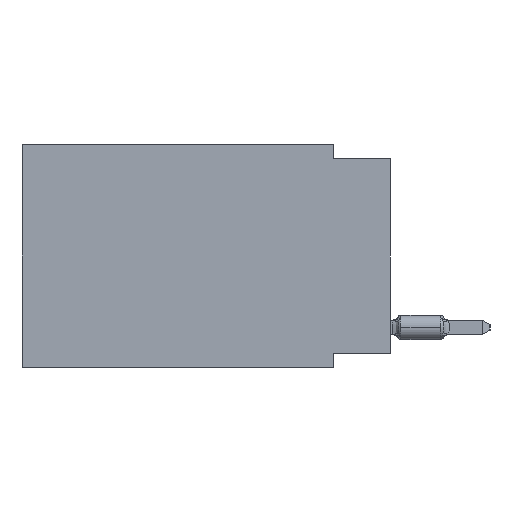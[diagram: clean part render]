
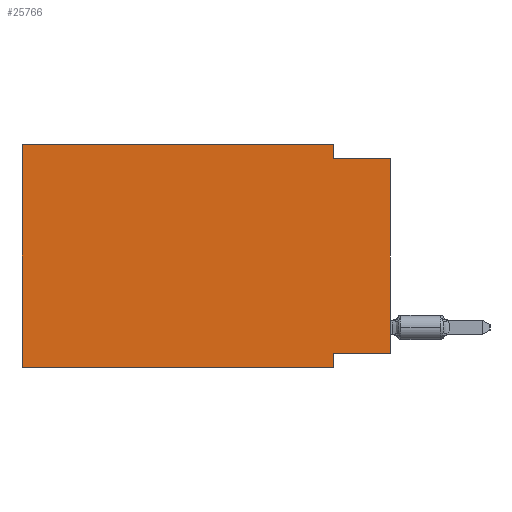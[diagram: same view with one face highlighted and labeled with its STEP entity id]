
A CAD part, left-side view. The second image highlights one B-rep face of the part: STEP entity #25766.
In plain terms, the highlighted planar face has unit normal (-1, 0, 0).
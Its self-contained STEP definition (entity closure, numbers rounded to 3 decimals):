
#37 = EDGE_LOOP ( 'NONE', ( #18887, #51576, #53976, #53579, #916, #33754, #56700, #32716 ) ) ;
#266 = LINE ( 'NONE', #39104, #40673 ) ;
#916 = ORIENTED_EDGE ( 'NONE', *, *, #35793, .F. ) ;
#3983 = CARTESIAN_POINT ( 'NONE',  ( 0., 2.54, -9.271 ) ) ;
#4941 = CARTESIAN_POINT ( 'NONE',  ( 0., 16.383, 0. ) ) ;
#5141 = EDGE_CURVE ( 'NONE', #61657, #27286, #12565, .T. ) ;
#5491 = CARTESIAN_POINT ( 'NONE',  ( 0., 2.54, 0. ) ) ;
#6035 = DIRECTION ( 'NONE',  ( 0., 0., 1. ) ) ;
#6107 = LINE ( 'NONE', #60019, #44024 ) ;
#6186 = VERTEX_POINT ( 'NONE', #60438 ) ;
#7779 = DIRECTION ( 'NONE',  ( 0., 1., 0. ) ) ;
#9043 = CARTESIAN_POINT ( 'NONE',  ( 0., 2.54, 0. ) ) ;
#9535 = LINE ( 'NONE', #29086, #45503 ) ;
#11144 = DIRECTION ( 'NONE',  ( 0., 0., -1. ) ) ;
#11424 = VECTOR ( 'NONE', #50591, 1000. ) ;
#11545 = VERTEX_POINT ( 'NONE', #30824 ) ;
#11798 = VERTEX_POINT ( 'NONE', #18266 ) ;
#12565 = LINE ( 'NONE', #16747, #20380 ) ;
#12651 = AXIS2_PLACEMENT_3D ( 'NONE', #4941, #24484, #44091 ) ;
#14536 = FACE_OUTER_BOUND ( 'NONE', #37, .T. ) ;
#16324 = CARTESIAN_POINT ( 'NONE',  ( 0., 16.383, -9.906 ) ) ;
#16747 = CARTESIAN_POINT ( 'NONE',  ( 0., 0., -9.271 ) ) ;
#17463 = CARTESIAN_POINT ( 'NONE',  ( 0., 2.54, -9.906 ) ) ;
#18266 = CARTESIAN_POINT ( 'NONE',  ( 0., 0., -0.635 ) ) ;
#18365 = EDGE_CURVE ( 'NONE', #11545, #11798, #9535, .T. ) ;
#18887 = ORIENTED_EDGE ( 'NONE', *, *, #28869, .T. ) ;
#19659 = PLANE ( 'NONE',  #12651 ) ;
#20380 = VECTOR ( 'NONE', #7779, 1000. ) ;
#22411 = EDGE_CURVE ( 'NONE', #27286, #57413, #55450, .T. ) ;
#23155 = VECTOR ( 'NONE', #11144, 1000. ) ;
#24484 = DIRECTION ( 'NONE',  ( 1., 0., 0. ) ) ;
#25231 = CARTESIAN_POINT ( 'NONE',  ( 0., 16.383, 0. ) ) ;
#25766 = ADVANCED_FACE ( 'NONE', ( #14536 ), #19659, .F. ) ;
#26290 = EDGE_CURVE ( 'NONE', #6186, #57413, #60319, .T. ) ;
#27286 = VERTEX_POINT ( 'NONE', #3983 ) ;
#28869 = EDGE_CURVE ( 'NONE', #61657, #11798, #266, .T. ) ;
#29022 = CARTESIAN_POINT ( 'NONE',  ( 0., 0., -9.271 ) ) ;
#29086 = CARTESIAN_POINT ( 'NONE',  ( 0., 0., -0.635 ) ) ;
#30824 = CARTESIAN_POINT ( 'NONE',  ( 0., 2.54, -0.635 ) ) ;
#32716 = ORIENTED_EDGE ( 'NONE', *, *, #5141, .F. ) ;
#33537 = VECTOR ( 'NONE', #62321, 1000. ) ;
#33754 = ORIENTED_EDGE ( 'NONE', *, *, #26290, .T. ) ;
#33808 = VERTEX_POINT ( 'NONE', #25231 ) ;
#35793 = EDGE_CURVE ( 'NONE', #6186, #33808, #55408, .T. ) ;
#39104 = CARTESIAN_POINT ( 'NONE',  ( 0., 0., 0. ) ) ;
#39183 = DIRECTION ( 'NONE',  ( 0., -1., 0. ) ) ;
#40378 = CARTESIAN_POINT ( 'NONE',  ( 0., 2.54, -9.906 ) ) ;
#40403 = VECTOR ( 'NONE', #51016, 1000. ) ;
#40673 = VECTOR ( 'NONE', #6035, 1000. ) ;
#42755 = LINE ( 'NONE', #9043, #33537 ) ;
#44024 = VECTOR ( 'NONE', #39183, 1000. ) ;
#44091 = DIRECTION ( 'NONE',  ( 0., 0., -1. ) ) ;
#44249 = VERTEX_POINT ( 'NONE', #5491 ) ;
#45503 = VECTOR ( 'NONE', #48693, 1000. ) ;
#48693 = DIRECTION ( 'NONE',  ( 0., -1., 0. ) ) ;
#50370 = EDGE_CURVE ( 'NONE', #44249, #11545, #42755, .T. ) ;
#50591 = DIRECTION ( 'NONE',  ( 0., 0., 1. ) ) ;
#51016 = DIRECTION ( 'NONE',  ( 0., -1., 0. ) ) ;
#51576 = ORIENTED_EDGE ( 'NONE', *, *, #18365, .F. ) ;
#53258 = EDGE_CURVE ( 'NONE', #33808, #44249, #6107, .T. ) ;
#53579 = ORIENTED_EDGE ( 'NONE', *, *, #53258, .F. ) ;
#53976 = ORIENTED_EDGE ( 'NONE', *, *, #50370, .F. ) ;
#54469 = CARTESIAN_POINT ( 'NONE',  ( 0., 16.383, 0. ) ) ;
#55408 = LINE ( 'NONE', #54469, #11424 ) ;
#55450 = LINE ( 'NONE', #40378, #23155 ) ;
#56700 = ORIENTED_EDGE ( 'NONE', *, *, #22411, .F. ) ;
#57413 = VERTEX_POINT ( 'NONE', #17463 ) ;
#60019 = CARTESIAN_POINT ( 'NONE',  ( 0., 16.383, 0. ) ) ;
#60319 = LINE ( 'NONE', #16324, #40403 ) ;
#60438 = CARTESIAN_POINT ( 'NONE',  ( 0., 16.383, -9.906 ) ) ;
#61657 = VERTEX_POINT ( 'NONE', #29022 ) ;
#62321 = DIRECTION ( 'NONE',  ( 0., 0., -1. ) ) ;
